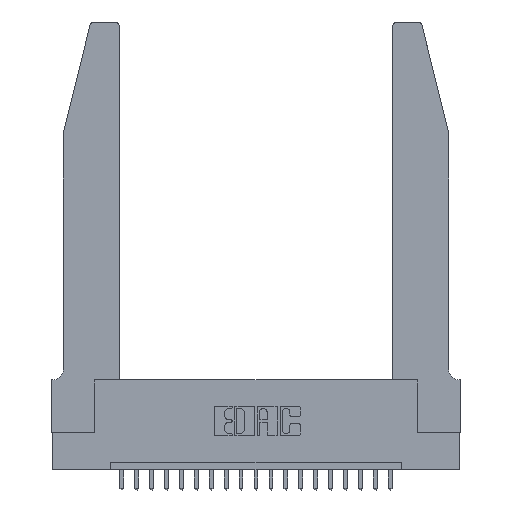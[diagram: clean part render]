
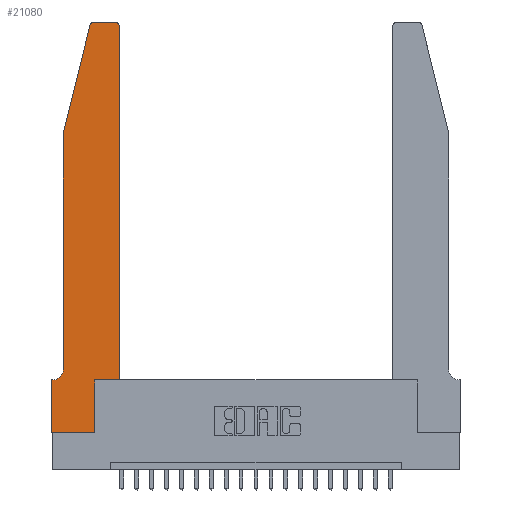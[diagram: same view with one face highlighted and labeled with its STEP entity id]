
A CAD part, top view. The second image highlights one B-rep face of the part: STEP entity #21080.
In plain terms, the highlighted planar face has unit normal (0, 0, 1).
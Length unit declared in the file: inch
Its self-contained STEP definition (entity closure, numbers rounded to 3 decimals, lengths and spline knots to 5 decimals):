
#335 = CARTESIAN_POINT ( 'NONE',  ( 0.284, 2.75, 0.37 ) ) ;
#577 = ORIENTED_EDGE ( 'NONE', *, *, #5270, .T. ) ;
#583 = CARTESIAN_POINT ( 'NONE',  ( 0.0055, 0.35, 0.37 ) ) ;
#626 = CARTESIAN_POINT ( 'NONE',  ( 0.0755, 2., 0.37 ) ) ;
#867 = CIRCLE ( 'NONE', #18093, 0.07 ) ;
#1132 = ORIENTED_EDGE ( 'NONE', *, *, #22191, .T. ) ;
#1348 = VECTOR ( 'NONE', #4207, 39.37008 ) ;
#1670 = DIRECTION ( 'NONE',  ( 0., 0., -1. ) ) ;
#1672 = ORIENTED_EDGE ( 'NONE', *, *, #20961, .T. ) ;
#1718 = CARTESIAN_POINT ( 'NONE',  ( 0.4505, 0.35, 0.37 ) ) ;
#2404 = VECTOR ( 'NONE', #18606, 39.37008 ) ;
#2659 = ORIENTED_EDGE ( 'NONE', *, *, #10819, .T. ) ;
#2893 = ORIENTED_EDGE ( 'NONE', *, *, #10964, .T. ) ;
#3265 = CARTESIAN_POINT ( 'NONE',  ( 0.4505, 0.35, 0.37 ) ) ;
#3288 = VECTOR ( 'NONE', #15489, 39.37008 ) ;
#3478 = DIRECTION ( 'NONE',  ( 0., -1., 0. ) ) ;
#3519 = LINE ( 'NONE', #12246, #18193 ) ;
#3529 = VERTEX_POINT ( 'NONE', #3827 ) ;
#3696 = CARTESIAN_POINT ( 'NONE',  ( 0.0755, 2., 0.37 ) ) ;
#3721 = AXIS2_PLACEMENT_3D ( 'NONE', #18327, #4681, #19916 ) ;
#3827 = CARTESIAN_POINT ( 'NONE',  ( 0.2865, 0.35, 0.37 ) ) ;
#3950 = CARTESIAN_POINT ( 'NONE',  ( 0., 0.35, 0.37 ) ) ;
#4207 = DIRECTION ( 'NONE',  ( 0., -1., 0. ) ) ;
#4658 = CARTESIAN_POINT ( 'NONE',  ( 0.2605, 2.75, 0.37 ) ) ;
#4681 = DIRECTION ( 'NONE',  ( 0., 0., 1. ) ) ;
#5270 = EDGE_CURVE ( 'NONE', #18532, #8451, #14589, .T. ) ;
#5365 = FACE_OUTER_BOUND ( 'NONE', #17468, .T. ) ;
#6158 = LINE ( 'NONE', #9959, #12305 ) ;
#7245 = EDGE_CURVE ( 'NONE', #19773, #17275, #867, .T. ) ;
#7712 = CIRCLE ( 'NONE', #8060, 0.03 ) ;
#7827 = CARTESIAN_POINT ( 'NONE',  ( 0.4205, 2.75, 0.37 ) ) ;
#7923 = CARTESIAN_POINT ( 'NONE',  ( 0., 0.35, 0.37 ) ) ;
#8060 = AXIS2_PLACEMENT_3D ( 'NONE', #9439, #17710, #12491 ) ;
#8146 = VERTEX_POINT ( 'NONE', #335 ) ;
#8344 = EDGE_CURVE ( 'NONE', #13864, #14029, #21699, .T. ) ;
#8451 = VERTEX_POINT ( 'NONE', #17212 ) ;
#9055 = EDGE_CURVE ( 'NONE', #8451, #3529, #3519, .T. ) ;
#9093 = CARTESIAN_POINT ( 'NONE',  ( 0.25487, 2.72718, 0.37 ) ) ;
#9427 = PLANE ( 'NONE',  #19392 ) ;
#9439 = CARTESIAN_POINT ( 'NONE',  ( 0.284, 2.72, 0.37 ) ) ;
#9666 = ORIENTED_EDGE ( 'NONE', *, *, #21261, .T. ) ;
#9959 = CARTESIAN_POINT ( 'NONE',  ( 0.0755, 2., 0.37 ) ) ;
#10819 = EDGE_CURVE ( 'NONE', #16563, #8146, #12293, .T. ) ;
#10923 = LINE ( 'NONE', #3696, #15475 ) ;
#10964 = EDGE_CURVE ( 'NONE', #3529, #13864, #19792, .T. ) ;
#11114 = EDGE_CURVE ( 'NONE', #19497, #19773, #10923, .T. ) ;
#11355 = DIRECTION ( 'NONE',  ( -0.239, -0.971, 0. ) ) ;
#11482 = VECTOR ( 'NONE', #19908, 39.37008 ) ;
#11556 = ORIENTED_EDGE ( 'NONE', *, *, #11114, .T. ) ;
#11920 = DIRECTION ( 'NONE',  ( -1., 0., 0. ) ) ;
#12246 = CARTESIAN_POINT ( 'NONE',  ( 0.2865, 0.35, 0.37 ) ) ;
#12249 = ORIENTED_EDGE ( 'NONE', *, *, #9055, .T. ) ;
#12293 = LINE ( 'NONE', #4658, #11482 ) ;
#12305 = VECTOR ( 'NONE', #11355, 39.37008 ) ;
#12443 = ORIENTED_EDGE ( 'NONE', *, *, #7245, .T. ) ;
#12451 = CIRCLE ( 'NONE', #3721, 0.03 ) ;
#12491 = DIRECTION ( 'NONE',  ( 1., 0., 0. ) ) ;
#12780 = CARTESIAN_POINT ( 'NONE',  ( 0., 0., 0.37 ) ) ;
#12969 = EDGE_CURVE ( 'NONE', #14029, #16563, #12451, .T. ) ;
#13224 = DIRECTION ( 'NONE',  ( 1., 0., 0. ) ) ;
#13864 = VERTEX_POINT ( 'NONE', #22181 ) ;
#14029 = VERTEX_POINT ( 'NONE', #15263 ) ;
#14589 = LINE ( 'NONE', #18329, #15663 ) ;
#15263 = CARTESIAN_POINT ( 'NONE',  ( 0.4505, 2.72, 0.37 ) ) ;
#15271 = LINE ( 'NONE', #12780, #1348 ) ;
#15475 = VECTOR ( 'NONE', #3478, 39.37008 ) ;
#15489 = DIRECTION ( 'NONE',  ( 0., 1., 0. ) ) ;
#15663 = VECTOR ( 'NONE', #21701, 39.37008 ) ;
#16085 = VECTOR ( 'NONE', #18581, 39.37008 ) ;
#16474 = DIRECTION ( 'NONE',  ( 0., 1., 0. ) ) ;
#16563 = VERTEX_POINT ( 'NONE', #7827 ) ;
#16614 = ORIENTED_EDGE ( 'NONE', *, *, #8344, .T. ) ;
#16754 = EDGE_CURVE ( 'NONE', #8146, #20458, #7712, .T. ) ;
#17088 = CARTESIAN_POINT ( 'NONE',  ( 0.0055, 0.42, 0.37 ) ) ;
#17212 = CARTESIAN_POINT ( 'NONE',  ( 0.2865, 0., 0.37 ) ) ;
#17275 = VERTEX_POINT ( 'NONE', #583 ) ;
#17468 = EDGE_LOOP ( 'NONE', ( #2659, #20412, #1132, #11556, #12443, #9666, #1672, #577, #12249, #2893, #16614, #18218 ) ) ;
#17710 = DIRECTION ( 'NONE',  ( 0., 0., 1. ) ) ;
#18093 = AXIS2_PLACEMENT_3D ( 'NONE', #17088, #1670, #11920 ) ;
#18193 = VECTOR ( 'NONE', #16474, 39.37008 ) ;
#18218 = ORIENTED_EDGE ( 'NONE', *, *, #12969, .T. ) ;
#18327 = CARTESIAN_POINT ( 'NONE',  ( 0.4205, 2.72, 0.37 ) ) ;
#18329 = CARTESIAN_POINT ( 'NONE',  ( 0., 0., 0.37 ) ) ;
#18532 = VERTEX_POINT ( 'NONE', #19051 ) ;
#18581 = DIRECTION ( 'NONE',  ( -1., 0., 0. ) ) ;
#18606 = DIRECTION ( 'NONE',  ( 1., 0., 0. ) ) ;
#18877 = VERTEX_POINT ( 'NONE', #3950 ) ;
#19051 = CARTESIAN_POINT ( 'NONE',  ( 0., 0., 0.37 ) ) ;
#19392 = AXIS2_PLACEMENT_3D ( 'NONE', #7923, #21455, #13224 ) ;
#19490 = CARTESIAN_POINT ( 'NONE',  ( 0.0755, 0.42, 0.37 ) ) ;
#19497 = VERTEX_POINT ( 'NONE', #626 ) ;
#19773 = VERTEX_POINT ( 'NONE', #19490 ) ;
#19792 = LINE ( 'NONE', #3265, #2404 ) ;
#19908 = DIRECTION ( 'NONE',  ( -1., 0., 0. ) ) ;
#19916 = DIRECTION ( 'NONE',  ( 1., 0., 0. ) ) ;
#20382 = CARTESIAN_POINT ( 'NONE',  ( 0.0755, 0.35, 0.37 ) ) ;
#20412 = ORIENTED_EDGE ( 'NONE', *, *, #16754, .T. ) ;
#20458 = VERTEX_POINT ( 'NONE', #9093 ) ;
#20659 = LINE ( 'NONE', #20382, #16085 ) ;
#20961 = EDGE_CURVE ( 'NONE', #18877, #18532, #15271, .T. ) ;
#21080 = ADVANCED_FACE ( 'NONE', ( #5365 ), #9427, .T. ) ;
#21261 = EDGE_CURVE ( 'NONE', #17275, #18877, #20659, .T. ) ;
#21455 = DIRECTION ( 'NONE',  ( 0., 0., 1. ) ) ;
#21699 = LINE ( 'NONE', #1718, #3288 ) ;
#21701 = DIRECTION ( 'NONE',  ( 1., 0., 0. ) ) ;
#22181 = CARTESIAN_POINT ( 'NONE',  ( 0.4505, 0.35, 0.37 ) ) ;
#22191 = EDGE_CURVE ( 'NONE', #20458, #19497, #6158, .T. ) ;
